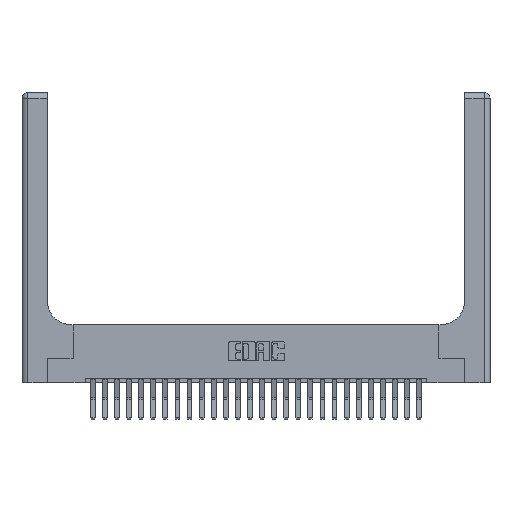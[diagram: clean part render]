
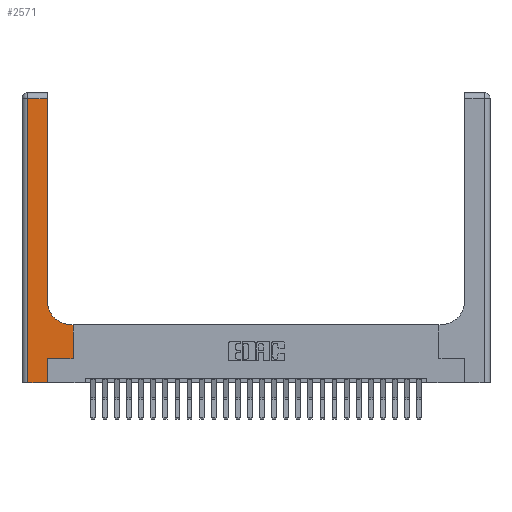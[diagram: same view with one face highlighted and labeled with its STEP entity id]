
A CAD part, top view. The second image highlights one B-rep face of the part: STEP entity #2571.
In plain terms, the highlighted planar face has unit normal (0, 0, 1).
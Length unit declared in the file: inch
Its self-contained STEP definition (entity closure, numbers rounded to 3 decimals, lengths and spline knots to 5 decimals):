
#281 = DIRECTION ( 'NONE',  ( 1., 0., 0. ) ) ;
#938 = EDGE_CURVE ( 'NONE', #8628, #22169, #2150, .T. ) ;
#1063 = VECTOR ( 'NONE', #14524, 39.37008 ) ;
#1081 = ORIENTED_EDGE ( 'NONE', *, *, #14375, .T. ) ;
#1590 = VERTEX_POINT ( 'NONE', #11090 ) ;
#1777 = DIRECTION ( 'NONE',  ( 0., -1., 0. ) ) ;
#2150 = LINE ( 'NONE', #19847, #24196 ) ;
#2571 = ADVANCED_FACE ( 'NONE', ( #24941 ), #25083, .F. ) ;
#2596 = CARTESIAN_POINT ( 'NONE',  ( 0.528, 0.25, 0.37 ) ) ;
#3242 = ORIENTED_EDGE ( 'NONE', *, *, #15819, .T. ) ;
#3589 = EDGE_CURVE ( 'NONE', #1590, #24299, #25408, .T. ) ;
#3768 = CARTESIAN_POINT ( 'NONE',  ( 0.26, 2.94, 0.37 ) ) ;
#4095 = CARTESIAN_POINT ( 'NONE',  ( 0.265, 0., 0.37 ) ) ;
#4595 = AXIS2_PLACEMENT_3D ( 'NONE', #11734, #15764, #14047 ) ;
#5053 = ORIENTED_EDGE ( 'NONE', *, *, #11335, .T. ) ;
#6322 = ORIENTED_EDGE ( 'NONE', *, *, #24224, .T. ) ;
#6338 = CARTESIAN_POINT ( 'NONE',  ( 0.26, 0.6, 0.37 ) ) ;
#6806 = VECTOR ( 'NONE', #9340, 39.37008 ) ;
#6947 = LINE ( 'NONE', #19275, #24458 ) ;
#7093 = VERTEX_POINT ( 'NONE', #3768 ) ;
#7230 = CARTESIAN_POINT ( 'NONE',  ( 0.06, 2.94, 0.37 ) ) ;
#7334 = DIRECTION ( 'NONE',  ( -1., 0., 0. ) ) ;
#7582 = EDGE_CURVE ( 'NONE', #24299, #15214, #11123, .T. ) ;
#8026 = EDGE_LOOP ( 'NONE', ( #5053, #25397, #17195, #3242, #1081, #17176, #10720, #22509, #6322 ) ) ;
#8288 = DIRECTION ( 'NONE',  ( -1., 0., 0. ) ) ;
#8579 = CARTESIAN_POINT ( 'NONE',  ( 0., 3., 0.37 ) ) ;
#8628 = VERTEX_POINT ( 'NONE', #7230 ) ;
#8656 = VERTEX_POINT ( 'NONE', #13398 ) ;
#8846 = EDGE_CURVE ( 'NONE', #15214, #8656, #20842, .T. ) ;
#9340 = DIRECTION ( 'NONE',  ( 0., 1., 0. ) ) ;
#10720 = ORIENTED_EDGE ( 'NONE', *, *, #7582, .T. ) ;
#10942 = DIRECTION ( 'NONE',  ( -1., 0., 0. ) ) ;
#11003 = DIRECTION ( 'NONE',  ( 1., 0., 0. ) ) ;
#11090 = CARTESIAN_POINT ( 'NONE',  ( 0.265, 0.25, 0.37 ) ) ;
#11123 = LINE ( 'NONE', #2596, #1063 ) ;
#11335 = EDGE_CURVE ( 'NONE', #20667, #7093, #14785, .T. ) ;
#11734 = CARTESIAN_POINT ( 'NONE',  ( 0.51, 0.85, 0.37 ) ) ;
#12865 = EDGE_CURVE ( 'NONE', #7093, #8628, #6947, .T. ) ;
#13331 = VECTOR ( 'NONE', #14539, 39.37008 ) ;
#13398 = CARTESIAN_POINT ( 'NONE',  ( 0.51, 0.6, 0.37 ) ) ;
#14047 = DIRECTION ( 'NONE',  ( 1., 0., 0. ) ) ;
#14375 = EDGE_CURVE ( 'NONE', #15934, #1590, #18587, .T. ) ;
#14524 = DIRECTION ( 'NONE',  ( 0., 1., 0. ) ) ;
#14539 = DIRECTION ( 'NONE',  ( 0., 1., 0. ) ) ;
#14784 = AXIS2_PLACEMENT_3D ( 'NONE', #8579, #24698, #10942 ) ;
#14785 = LINE ( 'NONE', #25298, #6806 ) ;
#15214 = VERTEX_POINT ( 'NONE', #23251 ) ;
#15764 = DIRECTION ( 'NONE',  ( 0., 0., -1. ) ) ;
#15819 = EDGE_CURVE ( 'NONE', #22169, #15934, #23759, .T. ) ;
#15934 = VERTEX_POINT ( 'NONE', #4095 ) ;
#15995 = CARTESIAN_POINT ( 'NONE',  ( 0., 0., 0.37 ) ) ;
#16379 = VECTOR ( 'NONE', #281, 39.37008 ) ;
#17176 = ORIENTED_EDGE ( 'NONE', *, *, #3589, .T. ) ;
#17195 = ORIENTED_EDGE ( 'NONE', *, *, #938, .T. ) ;
#18587 = LINE ( 'NONE', #22778, #13331 ) ;
#19275 = CARTESIAN_POINT ( 'NONE',  ( 0., 2.94, 0.37 ) ) ;
#19847 = CARTESIAN_POINT ( 'NONE',  ( 0.06, 3., 0.37 ) ) ;
#20286 = CARTESIAN_POINT ( 'NONE',  ( 0.06, 0., 0.37 ) ) ;
#20667 = VERTEX_POINT ( 'NONE', #20834 ) ;
#20834 = CARTESIAN_POINT ( 'NONE',  ( 0.26, 0.85, 0.37 ) ) ;
#20842 = LINE ( 'NONE', #6338, #21324 ) ;
#21324 = VECTOR ( 'NONE', #8288, 39.37008 ) ;
#21611 = CARTESIAN_POINT ( 'NONE',  ( 0.265, 0.25, 0.37 ) ) ;
#22169 = VERTEX_POINT ( 'NONE', #20286 ) ;
#22509 = ORIENTED_EDGE ( 'NONE', *, *, #8846, .T. ) ;
#22778 = CARTESIAN_POINT ( 'NONE',  ( 0.265, 0., 0.37 ) ) ;
#22827 = VECTOR ( 'NONE', #11003, 39.37008 ) ;
#23251 = CARTESIAN_POINT ( 'NONE',  ( 0.528, 0.6, 0.37 ) ) ;
#23759 = LINE ( 'NONE', #15995, #16379 ) ;
#24196 = VECTOR ( 'NONE', #1777, 39.37008 ) ;
#24224 = EDGE_CURVE ( 'NONE', #8656, #20667, #24685, .T. ) ;
#24299 = VERTEX_POINT ( 'NONE', #24677 ) ;
#24458 = VECTOR ( 'NONE', #7334, 39.37008 ) ;
#24677 = CARTESIAN_POINT ( 'NONE',  ( 0.528, 0.25, 0.37 ) ) ;
#24685 = CIRCLE ( 'NONE', #4595, 0.25 ) ;
#24698 = DIRECTION ( 'NONE',  ( 0., 0., -1. ) ) ;
#24941 = FACE_OUTER_BOUND ( 'NONE', #8026, .T. ) ;
#25083 = PLANE ( 'NONE',  #14784 ) ;
#25298 = CARTESIAN_POINT ( 'NONE',  ( 0.26, 3., 0.37 ) ) ;
#25397 = ORIENTED_EDGE ( 'NONE', *, *, #12865, .T. ) ;
#25408 = LINE ( 'NONE', #21611, #22827 ) ;
